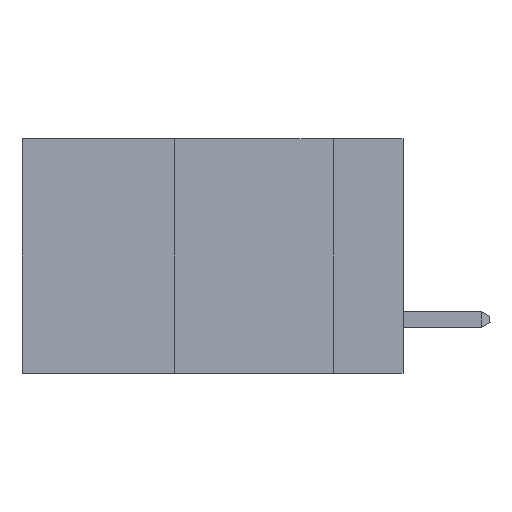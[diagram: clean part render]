
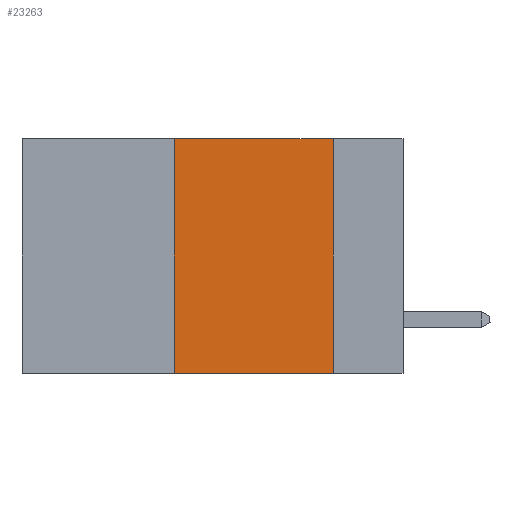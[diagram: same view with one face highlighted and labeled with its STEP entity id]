
A CAD part, left-side view. The second image highlights one B-rep face of the part: STEP entity #23263.
In plain terms, the highlighted planar face has unit normal (-1, 0, 0).
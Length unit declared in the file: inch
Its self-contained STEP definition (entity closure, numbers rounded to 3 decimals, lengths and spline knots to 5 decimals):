
#552 = DIRECTION ( 'NONE',  ( 0., 0., 1. ) ) ;
#1333 = DIRECTION ( 'NONE',  ( 0., -1., 0. ) ) ;
#2195 = VECTOR ( 'NONE', #552, 39.37008 ) ;
#2724 = CARTESIAN_POINT ( 'NONE',  ( 0., 0.36, -0.37 ) ) ;
#4078 = CARTESIAN_POINT ( 'NONE',  ( 0., 0.36, 0. ) ) ;
#5273 = EDGE_LOOP ( 'NONE', ( #31634, #30003, #17358, #40066 ) ) ;
#5432 = VERTEX_POINT ( 'NONE', #24498 ) ;
#6868 = VECTOR ( 'NONE', #25969, 39.37008 ) ;
#9511 = EDGE_CURVE ( 'NONE', #43313, #21014, #31607, .T. ) ;
#12560 = VECTOR ( 'NONE', #26927, 39.37008 ) ;
#17266 = LINE ( 'NONE', #30584, #12560 ) ;
#17358 = ORIENTED_EDGE ( 'NONE', *, *, #9511, .F. ) ;
#17651 = EDGE_CURVE ( 'NONE', #20694, #5432, #17266, .T. ) ;
#18902 = CARTESIAN_POINT ( 'NONE',  ( 0., 0.11, 0. ) ) ;
#20694 = VERTEX_POINT ( 'NONE', #18902 ) ;
#21014 = VERTEX_POINT ( 'NONE', #40300 ) ;
#22897 = CARTESIAN_POINT ( 'NONE',  ( 0., 0.6, 0. ) ) ;
#23019 = VECTOR ( 'NONE', #1333, 39.37008 ) ;
#23263 = ADVANCED_FACE ( 'NONE', ( #23389 ), #30256, .F. ) ;
#23389 = FACE_OUTER_BOUND ( 'NONE', #5273, .T. ) ;
#24498 = CARTESIAN_POINT ( 'NONE',  ( 0., 0.11, -0.37 ) ) ;
#24547 = LINE ( 'NONE', #35101, #23019 ) ;
#25969 = DIRECTION ( 'NONE',  ( 0., -1., 0. ) ) ;
#26845 = LINE ( 'NONE', #22897, #6868 ) ;
#26927 = DIRECTION ( 'NONE',  ( 0., 0., -1. ) ) ;
#27008 = CARTESIAN_POINT ( 'NONE',  ( 0., 0.6, 0. ) ) ;
#27969 = EDGE_CURVE ( 'NONE', #43313, #5432, #24547, .T. ) ;
#28346 = AXIS2_PLACEMENT_3D ( 'NONE', #27008, #36829, #33857 ) ;
#30003 = ORIENTED_EDGE ( 'NONE', *, *, #36506, .F. ) ;
#30256 = PLANE ( 'NONE',  #28346 ) ;
#30584 = CARTESIAN_POINT ( 'NONE',  ( 0., 0.11, 0. ) ) ;
#31607 = LINE ( 'NONE', #4078, #2195 ) ;
#31634 = ORIENTED_EDGE ( 'NONE', *, *, #17651, .F. ) ;
#33857 = DIRECTION ( 'NONE',  ( 0., 0., -1. ) ) ;
#35101 = CARTESIAN_POINT ( 'NONE',  ( 0., 0.6, -0.37 ) ) ;
#36506 = EDGE_CURVE ( 'NONE', #21014, #20694, #26845, .T. ) ;
#36829 = DIRECTION ( 'NONE',  ( 1., 0., 0. ) ) ;
#40066 = ORIENTED_EDGE ( 'NONE', *, *, #27969, .T. ) ;
#40300 = CARTESIAN_POINT ( 'NONE',  ( 0., 0.36, 0. ) ) ;
#43313 = VERTEX_POINT ( 'NONE', #2724 ) ;
